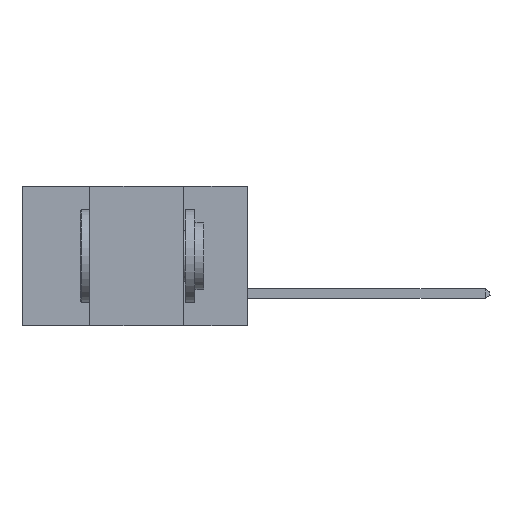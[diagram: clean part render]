
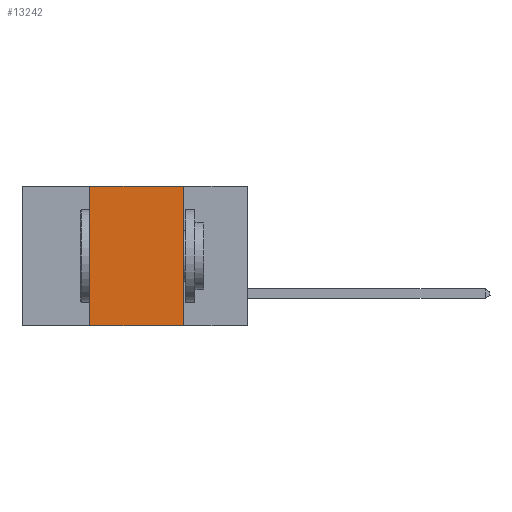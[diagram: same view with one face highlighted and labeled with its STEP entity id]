
A CAD part, left-side view. The second image highlights one B-rep face of the part: STEP entity #13242.
In plain terms, the highlighted planar face has unit normal (-1, 0, 0).
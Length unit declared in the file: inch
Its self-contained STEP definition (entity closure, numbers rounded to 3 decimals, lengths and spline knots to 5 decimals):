
#24 = LINE ( 'NONE', #12181, #16629 ) ;
#260 = VERTEX_POINT ( 'NONE', #492 ) ;
#492 = CARTESIAN_POINT ( 'NONE',  ( 0., 0.17, -0.37 ) ) ;
#1502 = PLANE ( 'NONE',  #14449 ) ;
#2942 = EDGE_CURVE ( 'NONE', #7015, #260, #9641, .T. ) ;
#3211 = VECTOR ( 'NONE', #10598, 39.37008 ) ;
#3216 = VERTEX_POINT ( 'NONE', #13581 ) ;
#3325 = VERTEX_POINT ( 'NONE', #14531 ) ;
#4953 = LINE ( 'NONE', #16254, #10947 ) ;
#6135 = DIRECTION ( 'NONE',  ( 0., 0., -1. ) ) ;
#6144 = VECTOR ( 'NONE', #12214, 39.37008 ) ;
#6441 = DIRECTION ( 'NONE',  ( 0., -1., 0. ) ) ;
#7015 = VERTEX_POINT ( 'NONE', #18695 ) ;
#7370 = ORIENTED_EDGE ( 'NONE', *, *, #15222, .F. ) ;
#7610 = CARTESIAN_POINT ( 'NONE',  ( 0., 0.6, 0. ) ) ;
#9641 = LINE ( 'NONE', #14153, #3211 ) ;
#10454 = DIRECTION ( 'NONE',  ( 0., -1., 0. ) ) ;
#10598 = DIRECTION ( 'NONE',  ( 0., 0., -1. ) ) ;
#10947 = VECTOR ( 'NONE', #10454, 39.37008 ) ;
#12181 = CARTESIAN_POINT ( 'NONE',  ( 0., 0.6, -0.37 ) ) ;
#12214 = DIRECTION ( 'NONE',  ( 0., 0., 1. ) ) ;
#12705 = ORIENTED_EDGE ( 'NONE', *, *, #17497, .T. ) ;
#12934 = ORIENTED_EDGE ( 'NONE', *, *, #2942, .F. ) ;
#13242 = ADVANCED_FACE ( 'NONE', ( #18664 ), #1502, .F. ) ;
#13561 = EDGE_LOOP ( 'NONE', ( #12934, #7370, #19057, #12705 ) ) ;
#13581 = CARTESIAN_POINT ( 'NONE',  ( 0., 0.42, 0. ) ) ;
#13681 = EDGE_CURVE ( 'NONE', #3325, #3216, #13986, .T. ) ;
#13986 = LINE ( 'NONE', #18465, #6144 ) ;
#14153 = CARTESIAN_POINT ( 'NONE',  ( 0., 0.17, 0. ) ) ;
#14449 = AXIS2_PLACEMENT_3D ( 'NONE', #7610, #14809, #6135 ) ;
#14531 = CARTESIAN_POINT ( 'NONE',  ( 0., 0.42, -0.37 ) ) ;
#14809 = DIRECTION ( 'NONE',  ( 1., 0., 0. ) ) ;
#15222 = EDGE_CURVE ( 'NONE', #3216, #7015, #4953, .T. ) ;
#16254 = CARTESIAN_POINT ( 'NONE',  ( 0., 0.6, 0. ) ) ;
#16629 = VECTOR ( 'NONE', #6441, 39.37008 ) ;
#17497 = EDGE_CURVE ( 'NONE', #3325, #260, #24, .T. ) ;
#18465 = CARTESIAN_POINT ( 'NONE',  ( 0., 0.42, 0. ) ) ;
#18664 = FACE_OUTER_BOUND ( 'NONE', #13561, .T. ) ;
#18695 = CARTESIAN_POINT ( 'NONE',  ( 0., 0.17, 0. ) ) ;
#19057 = ORIENTED_EDGE ( 'NONE', *, *, #13681, .F. ) ;
